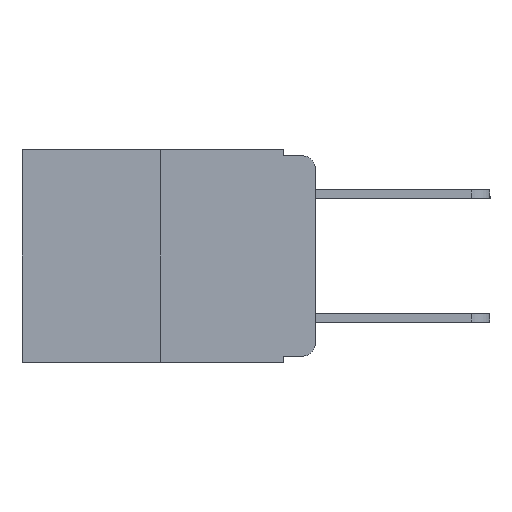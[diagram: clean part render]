
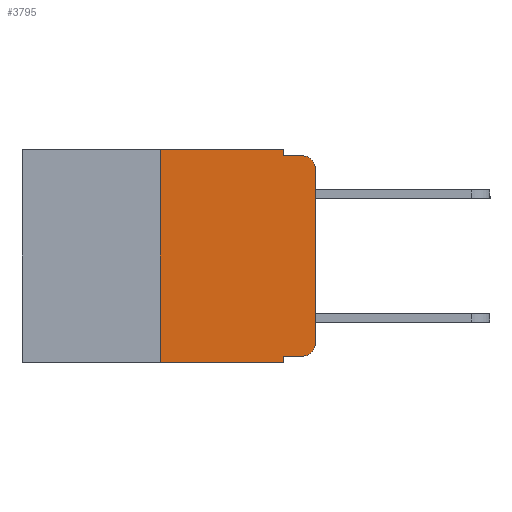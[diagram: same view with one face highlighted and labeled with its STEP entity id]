
A CAD part, left-side view. The second image highlights one B-rep face of the part: STEP entity #3795.
In plain terms, the highlighted planar face has unit normal (-1, 0, 0).
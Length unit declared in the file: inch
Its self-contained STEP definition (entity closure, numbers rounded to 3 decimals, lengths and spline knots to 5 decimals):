
#14 = DIRECTION ( 'NONE',  ( 0., -1., 0. ) ) ;
#136 = CARTESIAN_POINT ( 'NONE',  ( 0., 0.051, -0.333 ) ) ;
#194 = VECTOR ( 'NONE', #11536, 39.37008 ) ;
#235 = ORIENTED_EDGE ( 'NONE', *, *, #17418, .T. ) ;
#452 = ORIENTED_EDGE ( 'NONE', *, *, #540, .F. ) ;
#540 = EDGE_CURVE ( 'NONE', #17069, #9891, #14959, .T. ) ;
#781 = VERTEX_POINT ( 'NONE', #15296 ) ;
#1196 = EDGE_CURVE ( 'NONE', #4501, #17159, #6768, .T. ) ;
#1303 = ORIENTED_EDGE ( 'NONE', *, *, #7915, .F. ) ;
#1390 = ORIENTED_EDGE ( 'NONE', *, *, #18334, .T. ) ;
#1457 = CARTESIAN_POINT ( 'NONE',  ( 0., 0.473, 0. ) ) ;
#1507 = VECTOR ( 'NONE', #12527, 39.37008 ) ;
#1523 = DIRECTION ( 'NONE',  ( 1., 0., 0. ) ) ;
#1553 = EDGE_CURVE ( 'NONE', #6842, #4788, #4046, .T. ) ;
#1759 = CARTESIAN_POINT ( 'NONE',  ( 0., 0.02, -0.01 ) ) ;
#1761 = AXIS2_PLACEMENT_3D ( 'NONE', #1457, #1523, #12535 ) ;
#2273 = CARTESIAN_POINT ( 'NONE',  ( 0., 0.25, -0.343 ) ) ;
#2596 = ORIENTED_EDGE ( 'NONE', *, *, #16000, .T. ) ;
#2621 = CARTESIAN_POINT ( 'NONE',  ( 0., 0.473, -0.343 ) ) ;
#3095 = ORIENTED_EDGE ( 'NONE', *, *, #11775, .F. ) ;
#3152 = CARTESIAN_POINT ( 'NONE',  ( 0., 0.051, -0.01 ) ) ;
#3297 = DIRECTION ( 'NONE',  ( 0., -1., 0. ) ) ;
#3532 = FACE_OUTER_BOUND ( 'NONE', #9144, .T. ) ;
#3795 = ADVANCED_FACE ( 'NONE', ( #3532 ), #11015, .F. ) ;
#4046 = LINE ( 'NONE', #9158, #19534 ) ;
#4162 = CARTESIAN_POINT ( 'NONE',  ( 0., 0.051, 0. ) ) ;
#4501 = VERTEX_POINT ( 'NONE', #6534 ) ;
#4656 = CARTESIAN_POINT ( 'NONE',  ( 0., 0.02, -0.03 ) ) ;
#4788 = VERTEX_POINT ( 'NONE', #8872 ) ;
#4987 = CARTESIAN_POINT ( 'NONE',  ( 0., 0.051, -0.343 ) ) ;
#5268 = DIRECTION ( 'NONE',  ( -1., 0., 0. ) ) ;
#5623 = VERTEX_POINT ( 'NONE', #3152 ) ;
#5683 = CIRCLE ( 'NONE', #6665, 0.02 ) ;
#6051 = DIRECTION ( 'NONE',  ( 0., 0., -1. ) ) ;
#6181 = LINE ( 'NONE', #4162, #9834 ) ;
#6234 = DIRECTION ( 'NONE',  ( 0., 0., -1. ) ) ;
#6534 = CARTESIAN_POINT ( 'NONE',  ( 0., 0., -0.313 ) ) ;
#6665 = AXIS2_PLACEMENT_3D ( 'NONE', #4656, #15391, #6234 ) ;
#6768 = LINE ( 'NONE', #12581, #1507 ) ;
#6842 = VERTEX_POINT ( 'NONE', #2273 ) ;
#6914 = EDGE_CURVE ( 'NONE', #781, #5623, #6181, .T. ) ;
#7915 = EDGE_CURVE ( 'NONE', #5623, #12400, #16813, .T. ) ;
#8116 = CARTESIAN_POINT ( 'NONE',  ( 0., 0.051, -0.01 ) ) ;
#8309 = VERTEX_POINT ( 'NONE', #8845 ) ;
#8773 = ORIENTED_EDGE ( 'NONE', *, *, #1196, .T. ) ;
#8845 = CARTESIAN_POINT ( 'NONE',  ( 0., 0.02, -0.333 ) ) ;
#8872 = CARTESIAN_POINT ( 'NONE',  ( 0., 0.25, 0. ) ) ;
#9144 = EDGE_LOOP ( 'NONE', ( #8773, #12438, #1303, #12314, #3095, #18668, #2596, #452, #1390, #235 ) ) ;
#9158 = CARTESIAN_POINT ( 'NONE',  ( 0., 0.25, 0. ) ) ;
#9834 = VECTOR ( 'NONE', #16395, 39.37008 ) ;
#9891 = VERTEX_POINT ( 'NONE', #4987 ) ;
#9977 = CARTESIAN_POINT ( 'NONE',  ( 0., 0.473, 0. ) ) ;
#10296 = CARTESIAN_POINT ( 'NONE',  ( 0., 0.051, -0.333 ) ) ;
#10839 = VECTOR ( 'NONE', #12148, 39.37008 ) ;
#11015 = PLANE ( 'NONE',  #1761 ) ;
#11021 = AXIS2_PLACEMENT_3D ( 'NONE', #14527, #5268, #15989 ) ;
#11536 = DIRECTION ( 'NONE',  ( 0., -1., 0. ) ) ;
#11775 = EDGE_CURVE ( 'NONE', #4788, #781, #12738, .T. ) ;
#12125 = DIRECTION ( 'NONE',  ( 0., 0., 1. ) ) ;
#12148 = DIRECTION ( 'NONE',  ( 0., -1., 0. ) ) ;
#12314 = ORIENTED_EDGE ( 'NONE', *, *, #6914, .F. ) ;
#12400 = VERTEX_POINT ( 'NONE', #1759 ) ;
#12438 = ORIENTED_EDGE ( 'NONE', *, *, #16099, .T. ) ;
#12527 = DIRECTION ( 'NONE',  ( 0., 0., 1. ) ) ;
#12535 = DIRECTION ( 'NONE',  ( 0., 0., -1. ) ) ;
#12581 = CARTESIAN_POINT ( 'NONE',  ( 0., 0., 0. ) ) ;
#12738 = LINE ( 'NONE', #9977, #194 ) ;
#13371 = CIRCLE ( 'NONE', #11021, 0.02 ) ;
#13581 = CARTESIAN_POINT ( 'NONE',  ( 0., 0.051, 0. ) ) ;
#14527 = CARTESIAN_POINT ( 'NONE',  ( 0., 0.02, -0.313 ) ) ;
#14959 = LINE ( 'NONE', #13581, #18277 ) ;
#14985 = CARTESIAN_POINT ( 'NONE',  ( 0., 0., -0.03 ) ) ;
#15296 = CARTESIAN_POINT ( 'NONE',  ( 0., 0.051, 0. ) ) ;
#15391 = DIRECTION ( 'NONE',  ( -1., 0., 0. ) ) ;
#15989 = DIRECTION ( 'NONE',  ( 0., 0., -1. ) ) ;
#16000 = EDGE_CURVE ( 'NONE', #6842, #9891, #19036, .T. ) ;
#16099 = EDGE_CURVE ( 'NONE', #17159, #12400, #5683, .T. ) ;
#16395 = DIRECTION ( 'NONE',  ( 0., 0., -1. ) ) ;
#16618 = VECTOR ( 'NONE', #14, 39.37008 ) ;
#16813 = LINE ( 'NONE', #8116, #16618 ) ;
#17069 = VERTEX_POINT ( 'NONE', #10296 ) ;
#17159 = VERTEX_POINT ( 'NONE', #14985 ) ;
#17418 = EDGE_CURVE ( 'NONE', #8309, #4501, #13371, .T. ) ;
#18270 = VECTOR ( 'NONE', #3297, 39.37008 ) ;
#18277 = VECTOR ( 'NONE', #6051, 39.37008 ) ;
#18334 = EDGE_CURVE ( 'NONE', #17069, #8309, #18712, .T. ) ;
#18668 = ORIENTED_EDGE ( 'NONE', *, *, #1553, .F. ) ;
#18712 = LINE ( 'NONE', #136, #18270 ) ;
#19036 = LINE ( 'NONE', #2621, #10839 ) ;
#19534 = VECTOR ( 'NONE', #12125, 39.37008 ) ;
